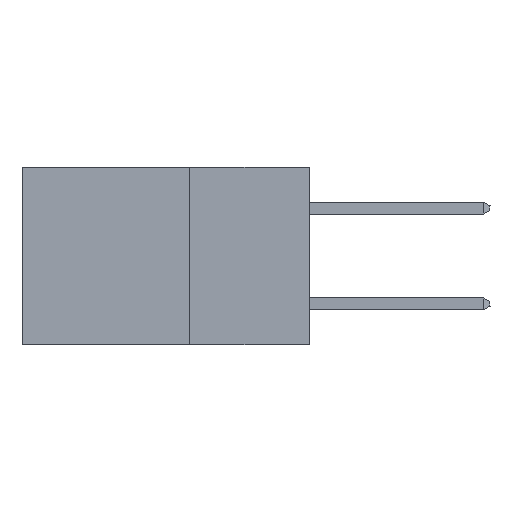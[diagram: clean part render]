
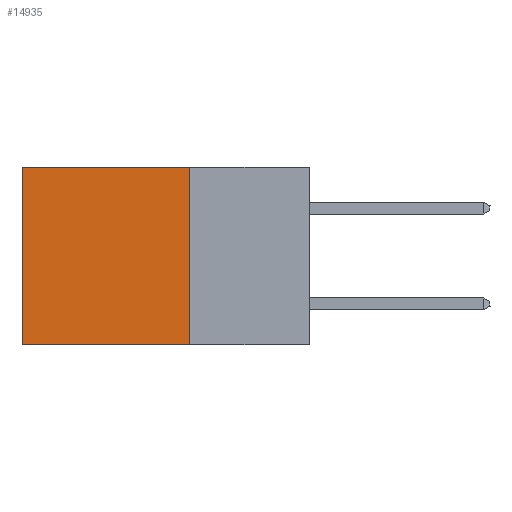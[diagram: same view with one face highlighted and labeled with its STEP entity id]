
A CAD part, left-side view. The second image highlights one B-rep face of the part: STEP entity #14935.
In plain terms, the highlighted planar face has unit normal (-1, 0, 0).
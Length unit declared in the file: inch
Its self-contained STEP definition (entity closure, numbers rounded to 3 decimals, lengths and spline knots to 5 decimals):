
#16 = DIRECTION ( 'NONE',  ( 0., 0., -1. ) ) ;
#152 = VECTOR ( 'NONE', #15656, 39.37008 ) ;
#547 = LINE ( 'NONE', #12748, #152 ) ;
#1153 = ORIENTED_EDGE ( 'NONE', *, *, #11068, .F. ) ;
#2287 = VERTEX_POINT ( 'NONE', #12367 ) ;
#2416 = LINE ( 'NONE', #14839, #14847 ) ;
#3122 = VERTEX_POINT ( 'NONE', #13115 ) ;
#3547 = LINE ( 'NONE', #14007, #7384 ) ;
#3840 = CARTESIAN_POINT ( 'NONE',  ( 0.2875, 0.25, 0. ) ) ;
#4234 = EDGE_CURVE ( 'NONE', #12132, #2287, #547, .T. ) ;
#4387 = CARTESIAN_POINT ( 'NONE',  ( 0.2875, 0.25, 0. ) ) ;
#5480 = ORIENTED_EDGE ( 'NONE', *, *, #4234, .T. ) ;
#6310 = DIRECTION ( 'NONE',  ( 0., 1., 0. ) ) ;
#7384 = VECTOR ( 'NONE', #7893, 39.37008 ) ;
#7657 = AXIS2_PLACEMENT_3D ( 'NONE', #12627, #7730, #16 ) ;
#7730 = DIRECTION ( 'NONE',  ( 1., 0., 0. ) ) ;
#7893 = DIRECTION ( 'NONE',  ( 0., 1., 0. ) ) ;
#9121 = VERTEX_POINT ( 'NONE', #3840 ) ;
#11068 = EDGE_CURVE ( 'NONE', #3122, #2287, #3547, .T. ) ;
#11761 = EDGE_LOOP ( 'NONE', ( #5480, #1153, #15020, #14858 ) ) ;
#11832 = VECTOR ( 'NONE', #14330, 39.37008 ) ;
#12010 = CARTESIAN_POINT ( 'NONE',  ( 0.2875, 0.6, 0. ) ) ;
#12132 = VERTEX_POINT ( 'NONE', #12010 ) ;
#12223 = LINE ( 'NONE', #4387, #11832 ) ;
#12367 = CARTESIAN_POINT ( 'NONE',  ( 0.2875, 0.6, -0.37 ) ) ;
#12528 = PLANE ( 'NONE',  #7657 ) ;
#12627 = CARTESIAN_POINT ( 'NONE',  ( 0.2875, 0.25, 0. ) ) ;
#12748 = CARTESIAN_POINT ( 'NONE',  ( 0.2875, 0.6, 0. ) ) ;
#13115 = CARTESIAN_POINT ( 'NONE',  ( 0.2875, 0.25, -0.37 ) ) ;
#13784 = FACE_OUTER_BOUND ( 'NONE', #11761, .T. ) ;
#14007 = CARTESIAN_POINT ( 'NONE',  ( 0.2875, 0.25, -0.37 ) ) ;
#14330 = DIRECTION ( 'NONE',  ( 0., 0., -1. ) ) ;
#14839 = CARTESIAN_POINT ( 'NONE',  ( 0.2875, 0.25, 0. ) ) ;
#14847 = VECTOR ( 'NONE', #6310, 39.37008 ) ;
#14858 = ORIENTED_EDGE ( 'NONE', *, *, #14867, .T. ) ;
#14867 = EDGE_CURVE ( 'NONE', #9121, #12132, #2416, .T. ) ;
#14935 = ADVANCED_FACE ( 'NONE', ( #13784 ), #12528, .F. ) ;
#15020 = ORIENTED_EDGE ( 'NONE', *, *, #15865, .F. ) ;
#15656 = DIRECTION ( 'NONE',  ( 0., 0., -1. ) ) ;
#15865 = EDGE_CURVE ( 'NONE', #9121, #3122, #12223, .T. ) ;
